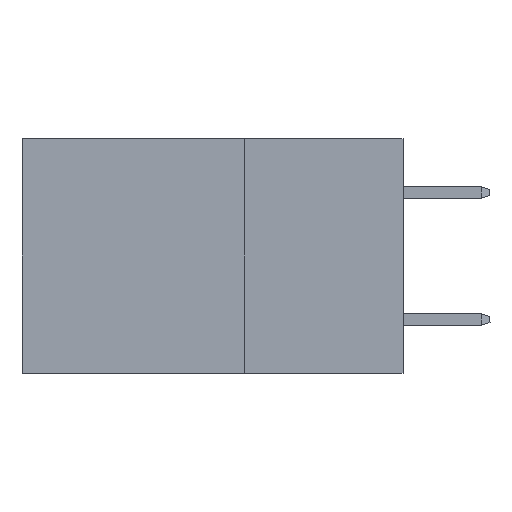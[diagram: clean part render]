
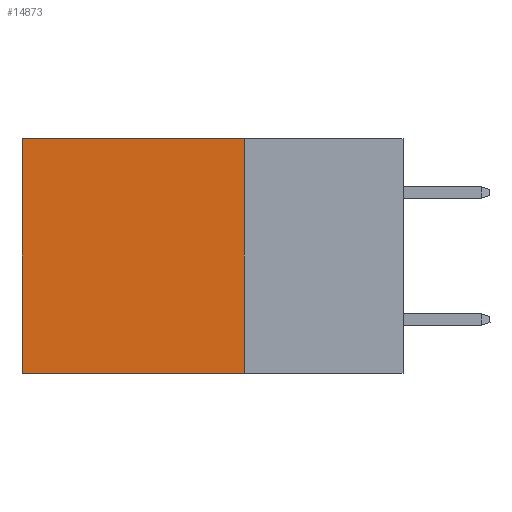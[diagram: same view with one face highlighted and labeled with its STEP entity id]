
A CAD part, left-side view. The second image highlights one B-rep face of the part: STEP entity #14873.
In plain terms, the highlighted planar face has unit normal (-1, 0, 0).
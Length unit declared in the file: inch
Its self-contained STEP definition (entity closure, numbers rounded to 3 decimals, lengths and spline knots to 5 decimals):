
#353 = LINE ( 'NONE', #5084, #11684 ) ;
#595 = VERTEX_POINT ( 'NONE', #10193 ) ;
#619 = EDGE_CURVE ( 'NONE', #5214, #9991, #353, .T. ) ;
#717 = ORIENTED_EDGE ( 'NONE', *, *, #12322, .T. ) ;
#1228 = LINE ( 'NONE', #12212, #6990 ) ;
#1727 = CARTESIAN_POINT ( 'NONE',  ( 0.2875, 0.25, 0. ) ) ;
#2244 = CARTESIAN_POINT ( 'NONE',  ( 0.2875, 0.25, 0. ) ) ;
#3157 = EDGE_CURVE ( 'NONE', #5214, #7709, #8487, .T. ) ;
#3327 = DIRECTION ( 'NONE',  ( 0., 0., -1. ) ) ;
#3924 = AXIS2_PLACEMENT_3D ( 'NONE', #1727, #7075, #3327 ) ;
#3972 = VECTOR ( 'NONE', #5118, 39.37008 ) ;
#4246 = CARTESIAN_POINT ( 'NONE',  ( 0.2875, 0.25, -0.37 ) ) ;
#4977 = DIRECTION ( 'NONE',  ( 0., 1., 0. ) ) ;
#5084 = CARTESIAN_POINT ( 'NONE',  ( 0.2875, 0.25, 0. ) ) ;
#5118 = DIRECTION ( 'NONE',  ( 0., 0., -1. ) ) ;
#5214 = VERTEX_POINT ( 'NONE', #2244 ) ;
#6362 = ORIENTED_EDGE ( 'NONE', *, *, #3157, .F. ) ;
#6990 = VECTOR ( 'NONE', #4977, 39.37008 ) ;
#7075 = DIRECTION ( 'NONE',  ( 1., 0., 0. ) ) ;
#7229 = CARTESIAN_POINT ( 'NONE',  ( 0.2875, 0.6, 0. ) ) ;
#7424 = CARTESIAN_POINT ( 'NONE',  ( 0.2875, 0.6, 0. ) ) ;
#7709 = VERTEX_POINT ( 'NONE', #4246 ) ;
#8487 = LINE ( 'NONE', #8575, #13951 ) ;
#8575 = CARTESIAN_POINT ( 'NONE',  ( 0.2875, 0.25, 0. ) ) ;
#8616 = LINE ( 'NONE', #7424, #3972 ) ;
#8877 = PLANE ( 'NONE',  #3924 ) ;
#9991 = VERTEX_POINT ( 'NONE', #7229 ) ;
#10193 = CARTESIAN_POINT ( 'NONE',  ( 0.2875, 0.6, -0.37 ) ) ;
#10347 = DIRECTION ( 'NONE',  ( 0., 1., 0. ) ) ;
#10981 = DIRECTION ( 'NONE',  ( 0., 0., -1. ) ) ;
#11684 = VECTOR ( 'NONE', #10347, 39.37008 ) ;
#12212 = CARTESIAN_POINT ( 'NONE',  ( 0.2875, 0.25, -0.37 ) ) ;
#12322 = EDGE_CURVE ( 'NONE', #9991, #595, #8616, .T. ) ;
#12334 = EDGE_CURVE ( 'NONE', #7709, #595, #1228, .T. ) ;
#13275 = ORIENTED_EDGE ( 'NONE', *, *, #12334, .F. ) ;
#13951 = VECTOR ( 'NONE', #10981, 39.37008 ) ;
#14347 = EDGE_LOOP ( 'NONE', ( #717, #13275, #6362, #15122 ) ) ;
#14830 = FACE_OUTER_BOUND ( 'NONE', #14347, .T. ) ;
#14873 = ADVANCED_FACE ( 'NONE', ( #14830 ), #8877, .F. ) ;
#15122 = ORIENTED_EDGE ( 'NONE', *, *, #619, .T. ) ;
